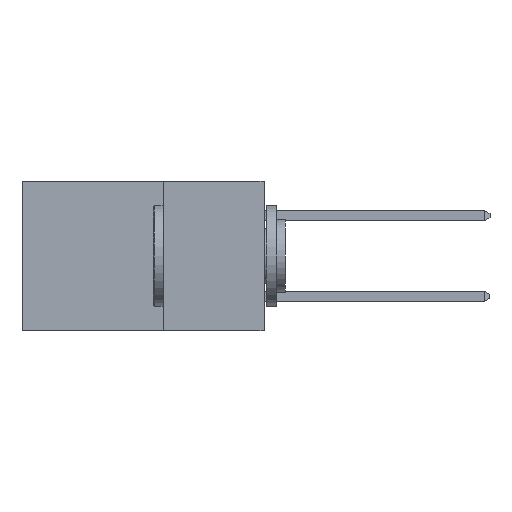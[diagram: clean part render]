
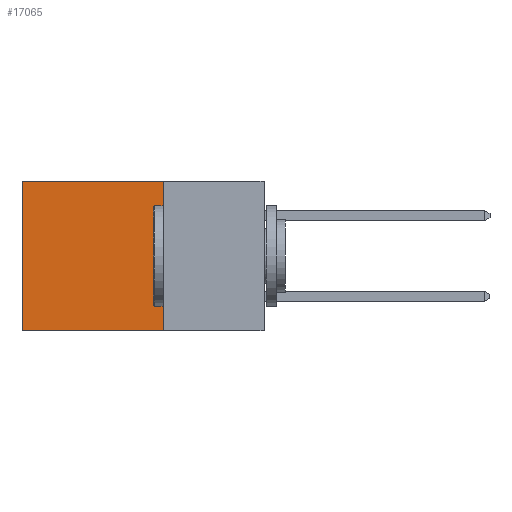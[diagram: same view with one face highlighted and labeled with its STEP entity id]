
A CAD part, left-side view. The second image highlights one B-rep face of the part: STEP entity #17065.
In plain terms, the highlighted planar face has unit normal (-1, 0, 0).
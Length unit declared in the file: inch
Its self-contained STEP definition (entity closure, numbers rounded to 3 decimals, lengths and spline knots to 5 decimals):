
#1127 = EDGE_CURVE ( 'NONE', #21511, #8845, #30800, .T. ) ;
#1783 = VECTOR ( 'NONE', #8569, 39.37008 ) ;
#2157 = VERTEX_POINT ( 'NONE', #9844 ) ;
#2388 = DIRECTION ( 'NONE',  ( 0., 0., -1. ) ) ;
#6021 = DIRECTION ( 'NONE',  ( 0., 1., 0. ) ) ;
#6164 = CARTESIAN_POINT ( 'NONE',  ( 0.298, 0.25, 0. ) ) ;
#6557 = CARTESIAN_POINT ( 'NONE',  ( 0.298, 0.6, 0. ) ) ;
#7907 = LINE ( 'NONE', #20255, #18498 ) ;
#8569 = DIRECTION ( 'NONE',  ( 0., 0., -1. ) ) ;
#8761 = EDGE_CURVE ( 'NONE', #2157, #21511, #7907, .T. ) ;
#8845 = VERTEX_POINT ( 'NONE', #25444 ) ;
#9610 = ORIENTED_EDGE ( 'NONE', *, *, #30332, .F. ) ;
#9675 = EDGE_LOOP ( 'NONE', ( #15019, #10080, #9610, #15351 ) ) ;
#9844 = CARTESIAN_POINT ( 'NONE',  ( 0.298, 0.25, 0. ) ) ;
#10080 = ORIENTED_EDGE ( 'NONE', *, *, #31035, .F. ) ;
#10681 = VERTEX_POINT ( 'NONE', #14426 ) ;
#11094 = DIRECTION ( 'NONE',  ( 0., 0., -1. ) ) ;
#11992 = CARTESIAN_POINT ( 'NONE',  ( 0.298, 0.25, 0. ) ) ;
#12261 = VECTOR ( 'NONE', #11094, 39.37008 ) ;
#14426 = CARTESIAN_POINT ( 'NONE',  ( 0.298, 0.25, -0.37 ) ) ;
#15019 = ORIENTED_EDGE ( 'NONE', *, *, #1127, .T. ) ;
#15351 = ORIENTED_EDGE ( 'NONE', *, *, #8761, .T. ) ;
#16417 = PLANE ( 'NONE',  #28426 ) ;
#16849 = DIRECTION ( 'NONE',  ( 1., 0., 0. ) ) ;
#17065 = ADVANCED_FACE ( 'NONE', ( #31102 ), #16417, .F. ) ;
#18498 = VECTOR ( 'NONE', #29962, 39.37008 ) ;
#20255 = CARTESIAN_POINT ( 'NONE',  ( 0.298, 0.25, 0. ) ) ;
#20497 = CARTESIAN_POINT ( 'NONE',  ( 0.298, 0.25, -0.37 ) ) ;
#20652 = LINE ( 'NONE', #20497, #21419 ) ;
#21419 = VECTOR ( 'NONE', #6021, 39.37008 ) ;
#21511 = VERTEX_POINT ( 'NONE', #23995 ) ;
#23995 = CARTESIAN_POINT ( 'NONE',  ( 0.298, 0.6, 0. ) ) ;
#25444 = CARTESIAN_POINT ( 'NONE',  ( 0.298, 0.6, -0.37 ) ) ;
#28264 = LINE ( 'NONE', #6164, #1783 ) ;
#28426 = AXIS2_PLACEMENT_3D ( 'NONE', #11992, #16849, #2388 ) ;
#29962 = DIRECTION ( 'NONE',  ( 0., 1., 0. ) ) ;
#30332 = EDGE_CURVE ( 'NONE', #2157, #10681, #28264, .T. ) ;
#30800 = LINE ( 'NONE', #6557, #12261 ) ;
#31035 = EDGE_CURVE ( 'NONE', #10681, #8845, #20652, .T. ) ;
#31102 = FACE_OUTER_BOUND ( 'NONE', #9675, .T. ) ;
